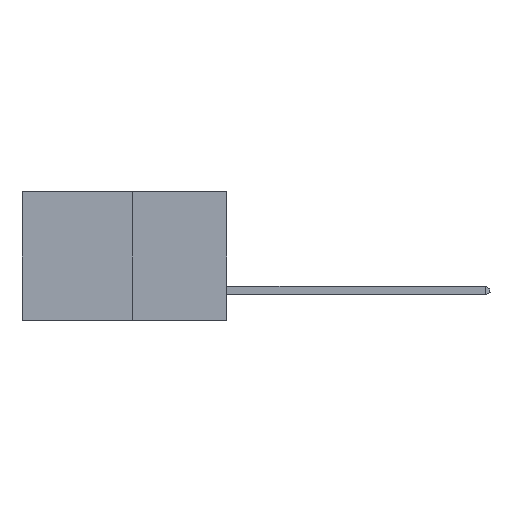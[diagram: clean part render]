
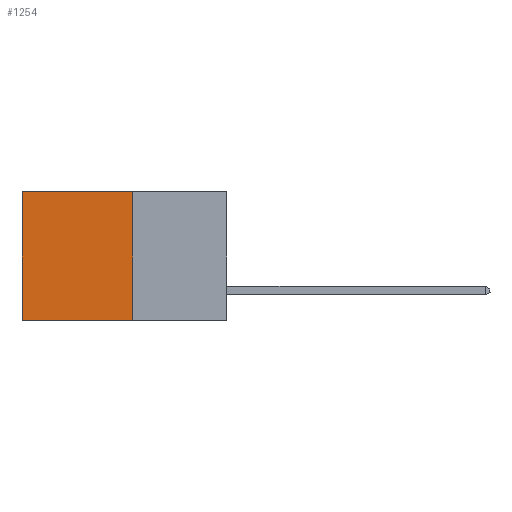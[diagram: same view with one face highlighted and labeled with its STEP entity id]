
A CAD part, left-side view. The second image highlights one B-rep face of the part: STEP entity #1254.
In plain terms, the highlighted planar face has unit normal (-1, 0, 0).
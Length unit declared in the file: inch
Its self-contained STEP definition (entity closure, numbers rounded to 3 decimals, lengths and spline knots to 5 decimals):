
#563 = LINE ( 'NONE', #9070, #20161 ) ;
#712 = EDGE_LOOP ( 'NONE', ( #2022, #2143, #2163, #2553 ) ) ;
#1241 = EDGE_CURVE ( 'NONE', #19312, #5234, #7816, .T. ) ;
#1254 = ADVANCED_FACE ( 'NONE', ( #19867 ), #18829, .F. ) ;
#2022 = ORIENTED_EDGE ( 'NONE', *, *, #1241, .T. ) ;
#2143 = ORIENTED_EDGE ( 'NONE', *, *, #17553, .F. ) ;
#2163 = ORIENTED_EDGE ( 'NONE', *, *, #13546, .F. ) ;
#2553 = ORIENTED_EDGE ( 'NONE', *, *, #7884, .T. ) ;
#3325 = CARTESIAN_POINT ( 'NONE',  ( 0.277, 0.27, 0. ) ) ;
#3586 = VECTOR ( 'NONE', #17585, 39.37008 ) ;
#4935 = VERTEX_POINT ( 'NONE', #15867 ) ;
#5234 = VERTEX_POINT ( 'NONE', #12759 ) ;
#5547 = CARTESIAN_POINT ( 'NONE',  ( 0.277, 0.27, -0.37 ) ) ;
#5566 = VECTOR ( 'NONE', #18135, 39.37008 ) ;
#6984 = VERTEX_POINT ( 'NONE', #3325 ) ;
#7816 = LINE ( 'NONE', #19450, #3586 ) ;
#7884 = EDGE_CURVE ( 'NONE', #6984, #19312, #19338, .T. ) ;
#9070 = CARTESIAN_POINT ( 'NONE',  ( 0.277, 0.27, -0.37 ) ) ;
#11007 = VECTOR ( 'NONE', #19332, 39.37008 ) ;
#12759 = CARTESIAN_POINT ( 'NONE',  ( 0.277, 0.59, -0.37 ) ) ;
#13546 = EDGE_CURVE ( 'NONE', #6984, #4935, #14038, .T. ) ;
#14038 = LINE ( 'NONE', #5547, #5566 ) ;
#15084 = CARTESIAN_POINT ( 'NONE',  ( 0.277, 0.59, 0. ) ) ;
#15234 = AXIS2_PLACEMENT_3D ( 'NONE', #15739, #19833, #19673 ) ;
#15431 = DIRECTION ( 'NONE',  ( 0., 1., 0. ) ) ;
#15739 = CARTESIAN_POINT ( 'NONE',  ( 0.277, 0.27, -0.37 ) ) ;
#15867 = CARTESIAN_POINT ( 'NONE',  ( 0.277, 0.27, -0.37 ) ) ;
#16267 = CARTESIAN_POINT ( 'NONE',  ( 0.277, 0.27, 0. ) ) ;
#17553 = EDGE_CURVE ( 'NONE', #4935, #5234, #563, .T. ) ;
#17585 = DIRECTION ( 'NONE',  ( 0., 0., -1. ) ) ;
#18135 = DIRECTION ( 'NONE',  ( 0., 0., -1. ) ) ;
#18829 = PLANE ( 'NONE',  #15234 ) ;
#19312 = VERTEX_POINT ( 'NONE', #15084 ) ;
#19332 = DIRECTION ( 'NONE',  ( 0., 1., 0. ) ) ;
#19338 = LINE ( 'NONE', #16267, #11007 ) ;
#19450 = CARTESIAN_POINT ( 'NONE',  ( 0.277, 0.59, -0.37 ) ) ;
#19673 = DIRECTION ( 'NONE',  ( 0., 0., -1. ) ) ;
#19833 = DIRECTION ( 'NONE',  ( 1., 0., 0. ) ) ;
#19867 = FACE_OUTER_BOUND ( 'NONE', #712, .T. ) ;
#20161 = VECTOR ( 'NONE', #15431, 39.37008 ) ;
